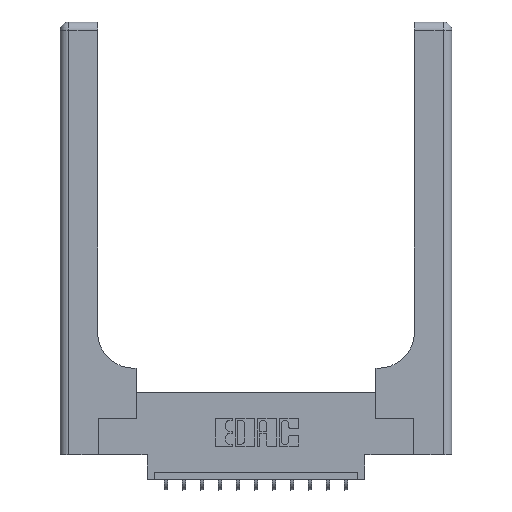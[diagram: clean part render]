
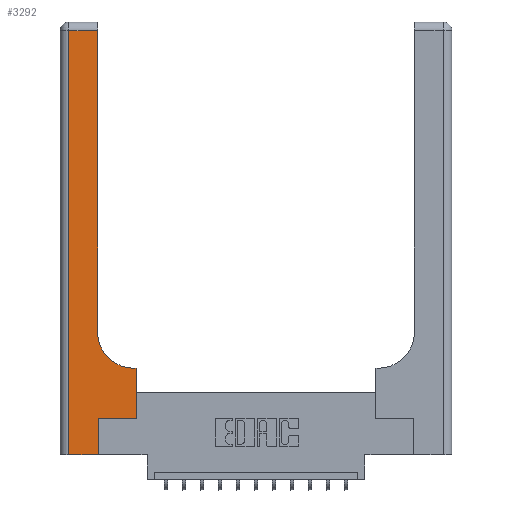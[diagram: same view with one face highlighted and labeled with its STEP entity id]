
A CAD part, top view. The second image highlights one B-rep face of the part: STEP entity #3292.
In plain terms, the highlighted planar face has unit normal (0, 0, 1).
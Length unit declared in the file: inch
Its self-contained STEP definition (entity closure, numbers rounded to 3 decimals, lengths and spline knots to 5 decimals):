
#329 = DIRECTION ( 'NONE',  ( 1., 0., 0. ) ) ;
#573 = LINE ( 'NONE', #14614, #6549 ) ;
#764 = CARTESIAN_POINT ( 'NONE',  ( 0., 2.94, 0.37 ) ) ;
#1132 = CARTESIAN_POINT ( 'NONE',  ( 0.26, 3., 0.37 ) ) ;
#1275 = ORIENTED_EDGE ( 'NONE', *, *, #10545, .T. ) ;
#1704 = CARTESIAN_POINT ( 'NONE',  ( 0.06, 3., 0.37 ) ) ;
#1866 = LINE ( 'NONE', #1704, #9181 ) ;
#2196 = EDGE_CURVE ( 'NONE', #16733, #14059, #8622, .T. ) ;
#2389 = FACE_OUTER_BOUND ( 'NONE', #5748, .T. ) ;
#2463 = DIRECTION ( 'NONE',  ( -1., 0., 0. ) ) ;
#2864 = CARTESIAN_POINT ( 'NONE',  ( 0.51, 0.6, 0.37 ) ) ;
#3292 = ADVANCED_FACE ( 'NONE', ( #2389 ), #3572, .F. ) ;
#3357 = EDGE_CURVE ( 'NONE', #15365, #14306, #11348, .T. ) ;
#3402 = CARTESIAN_POINT ( 'NONE',  ( 0., 3., 0.37 ) ) ;
#3572 = PLANE ( 'NONE',  #12698 ) ;
#4020 = VECTOR ( 'NONE', #16339, 39.37008 ) ;
#4168 = VERTEX_POINT ( 'NONE', #2864 ) ;
#5343 = CARTESIAN_POINT ( 'NONE',  ( 0.265, 0.25, 0.37 ) ) ;
#5491 = EDGE_CURVE ( 'NONE', #14063, #9634, #7797, .T. ) ;
#5552 = VECTOR ( 'NONE', #329, 39.37008 ) ;
#5632 = EDGE_CURVE ( 'NONE', #9634, #15365, #573, .T. ) ;
#5748 = EDGE_LOOP ( 'NONE', ( #12453, #11448, #1275, #11844, #7481, #8331, #6777, #7479, #11528 ) ) ;
#5844 = VECTOR ( 'NONE', #14478, 39.37008 ) ;
#6071 = EDGE_CURVE ( 'NONE', #4168, #16733, #12320, .T. ) ;
#6549 = VECTOR ( 'NONE', #6830, 39.37008 ) ;
#6777 = ORIENTED_EDGE ( 'NONE', *, *, #3357, .T. ) ;
#6830 = DIRECTION ( 'NONE',  ( 1., 0., 0. ) ) ;
#7016 = CARTESIAN_POINT ( 'NONE',  ( 0.528, 0.6, 0.37 ) ) ;
#7479 = ORIENTED_EDGE ( 'NONE', *, *, #12111, .T. ) ;
#7481 = ORIENTED_EDGE ( 'NONE', *, *, #5491, .T. ) ;
#7676 = AXIS2_PLACEMENT_3D ( 'NONE', #9221, #7953, #11960 ) ;
#7797 = LINE ( 'NONE', #9153, #15531 ) ;
#7953 = DIRECTION ( 'NONE',  ( 0., 0., -1. ) ) ;
#8331 = ORIENTED_EDGE ( 'NONE', *, *, #5632, .T. ) ;
#8622 = LINE ( 'NONE', #1132, #10955 ) ;
#8836 = LINE ( 'NONE', #764, #4020 ) ;
#9153 = CARTESIAN_POINT ( 'NONE',  ( 0.265, 0., 0.37 ) ) ;
#9181 = VECTOR ( 'NONE', #13380, 39.37008 ) ;
#9221 = CARTESIAN_POINT ( 'NONE',  ( 0.51, 0.85, 0.37 ) ) ;
#9385 = CARTESIAN_POINT ( 'NONE',  ( 0.265, 0., 0.37 ) ) ;
#9533 = CARTESIAN_POINT ( 'NONE',  ( 0., 0., 0.37 ) ) ;
#9634 = VERTEX_POINT ( 'NONE', #5343 ) ;
#9930 = EDGE_CURVE ( 'NONE', #14059, #14374, #8836, .T. ) ;
#10467 = CARTESIAN_POINT ( 'NONE',  ( 0.26, 0.6, 0.37 ) ) ;
#10545 = EDGE_CURVE ( 'NONE', #14374, #12172, #1866, .T. ) ;
#10955 = VECTOR ( 'NONE', #15003, 39.37008 ) ;
#11017 = EDGE_CURVE ( 'NONE', #12172, #14063, #15995, .T. ) ;
#11348 = LINE ( 'NONE', #12710, #5844 ) ;
#11448 = ORIENTED_EDGE ( 'NONE', *, *, #9930, .T. ) ;
#11528 = ORIENTED_EDGE ( 'NONE', *, *, #6071, .T. ) ;
#11752 = LINE ( 'NONE', #10467, #16202 ) ;
#11830 = CARTESIAN_POINT ( 'NONE',  ( 0.06, 0., 0.37 ) ) ;
#11844 = ORIENTED_EDGE ( 'NONE', *, *, #11017, .T. ) ;
#11960 = DIRECTION ( 'NONE',  ( 1., 0., 0. ) ) ;
#12111 = EDGE_CURVE ( 'NONE', #14306, #4168, #11752, .T. ) ;
#12172 = VERTEX_POINT ( 'NONE', #11830 ) ;
#12320 = CIRCLE ( 'NONE', #7676, 0.25 ) ;
#12453 = ORIENTED_EDGE ( 'NONE', *, *, #2196, .T. ) ;
#12495 = CARTESIAN_POINT ( 'NONE',  ( 0.06, 2.94, 0.37 ) ) ;
#12698 = AXIS2_PLACEMENT_3D ( 'NONE', #3402, #12796, #15001 ) ;
#12710 = CARTESIAN_POINT ( 'NONE',  ( 0.528, 0.25, 0.37 ) ) ;
#12796 = DIRECTION ( 'NONE',  ( 0., 0., -1. ) ) ;
#13380 = DIRECTION ( 'NONE',  ( 0., -1., 0. ) ) ;
#14059 = VERTEX_POINT ( 'NONE', #14579 ) ;
#14063 = VERTEX_POINT ( 'NONE', #9385 ) ;
#14306 = VERTEX_POINT ( 'NONE', #7016 ) ;
#14357 = DIRECTION ( 'NONE',  ( 0., 1., 0. ) ) ;
#14374 = VERTEX_POINT ( 'NONE', #12495 ) ;
#14373 = CARTESIAN_POINT ( 'NONE',  ( 0.528, 0.25, 0.37 ) ) ;
#14478 = DIRECTION ( 'NONE',  ( 0., 1., 0. ) ) ;
#14579 = CARTESIAN_POINT ( 'NONE',  ( 0.26, 2.94, 0.37 ) ) ;
#14614 = CARTESIAN_POINT ( 'NONE',  ( 0.265, 0.25, 0.37 ) ) ;
#14743 = CARTESIAN_POINT ( 'NONE',  ( 0.26, 0.85, 0.37 ) ) ;
#15001 = DIRECTION ( 'NONE',  ( -1., 0., 0. ) ) ;
#15003 = DIRECTION ( 'NONE',  ( 0., 1., 0. ) ) ;
#15365 = VERTEX_POINT ( 'NONE', #14373 ) ;
#15531 = VECTOR ( 'NONE', #14357, 39.37008 ) ;
#15995 = LINE ( 'NONE', #9533, #5552 ) ;
#16202 = VECTOR ( 'NONE', #2463, 39.37008 ) ;
#16339 = DIRECTION ( 'NONE',  ( -1., 0., 0. ) ) ;
#16733 = VERTEX_POINT ( 'NONE', #14743 ) ;
